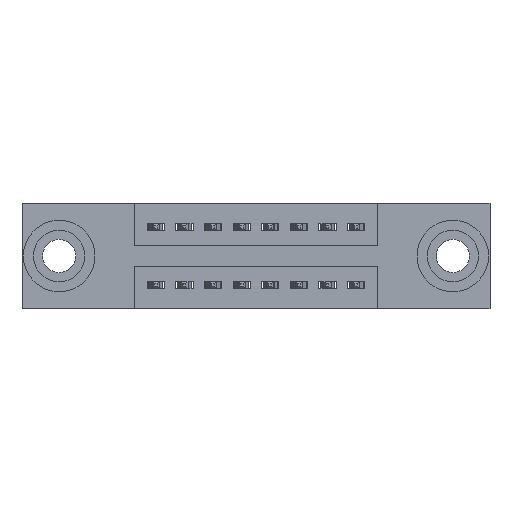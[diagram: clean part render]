
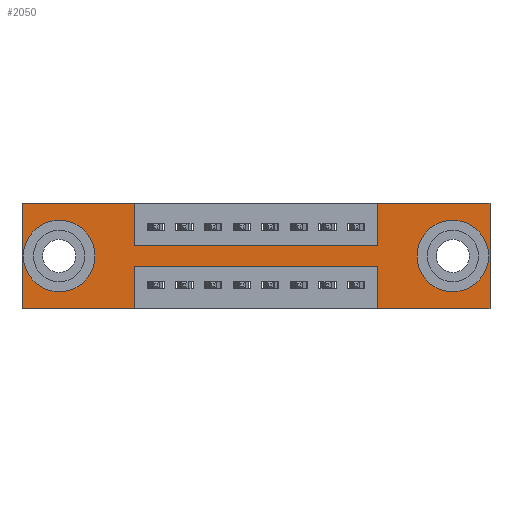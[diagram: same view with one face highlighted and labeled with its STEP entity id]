
A CAD part, front view. The second image highlights one B-rep face of the part: STEP entity #2050.
In plain terms, the highlighted planar face has unit normal (0, -1, 0).
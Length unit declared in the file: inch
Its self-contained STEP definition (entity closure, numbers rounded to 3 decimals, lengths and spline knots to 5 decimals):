
#73 = VERTEX_POINT ( 'NONE', #9574 ) ;
#88 = CARTESIAN_POINT ( 'NONE',  ( 0.13, 0., -0.263 ) ) ;
#96 = EDGE_CURVE ( 'NONE', #6298, #6497, #2246, .T. ) ;
#97 = CARTESIAN_POINT ( 'NONE',  ( 1.505, 0., -0.185 ) ) ;
#243 = EDGE_CURVE ( 'NONE', #3637, #3447, #795, .T. ) ;
#265 = VERTEX_POINT ( 'NONE', #3501 ) ;
#317 = EDGE_CURVE ( 'NONE', #73, #8299, #4881, .T. ) ;
#341 = AXIS2_PLACEMENT_3D ( 'NONE', #10581, #5446, #11437 ) ;
#378 = VERTEX_POINT ( 'NONE', #7372 ) ;
#380 = CIRCLE ( 'NONE', #341, 0.078 ) ;
#427 = EDGE_CURVE ( 'NONE', #7613, #6013, #10150, .T. ) ;
#436 = VECTOR ( 'NONE', #5695, 39.37008 ) ;
#519 = DIRECTION ( 'NONE',  ( 0., 0., -1. ) ) ;
#743 = LINE ( 'NONE', #5140, #436 ) ;
#795 = LINE ( 'NONE', #10824, #8054 ) ;
#910 = CIRCLE ( 'NONE', #2896, 0.078 ) ;
#936 = VECTOR ( 'NONE', #5049, 39.37008 ) ;
#1004 = AXIS2_PLACEMENT_3D ( 'NONE', #1729, #8076, #2676 ) ;
#1240 = ORIENTED_EDGE ( 'NONE', *, *, #7634, .F. ) ;
#1386 = ORIENTED_EDGE ( 'NONE', *, *, #8331, .T. ) ;
#1442 = CARTESIAN_POINT ( 'NONE',  ( 1.2425, 0., 0. ) ) ;
#1458 = LINE ( 'NONE', #6986, #8415 ) ;
#1478 = CIRCLE ( 'NONE', #1004, 0.078 ) ;
#1482 = DIRECTION ( 'NONE',  ( 0., 0., -1. ) ) ;
#1713 = EDGE_CURVE ( 'NONE', #10849, #4046, #7480, .T. ) ;
#1729 = CARTESIAN_POINT ( 'NONE',  ( 0.13, 0., -0.185 ) ) ;
#1845 = ORIENTED_EDGE ( 'NONE', *, *, #11431, .F. ) ;
#1887 = CARTESIAN_POINT ( 'NONE',  ( 0., 0., -0.37 ) ) ;
#1901 = CARTESIAN_POINT ( 'NONE',  ( 0.3925, 0., -0.22 ) ) ;
#2050 = ADVANCED_FACE ( 'NONE', ( #4439, #11041, #4976 ), #3816, .T. ) ;
#2130 = CARTESIAN_POINT ( 'NONE',  ( 1.2425, 0., -0.37 ) ) ;
#2155 = EDGE_CURVE ( 'NONE', #378, #265, #743, .T. ) ;
#2246 = LINE ( 'NONE', #6984, #6827 ) ;
#2374 = AXIS2_PLACEMENT_3D ( 'NONE', #97, #3207, #519 ) ;
#2391 = DIRECTION ( 'NONE',  ( 0., 0., 1. ) ) ;
#2406 = ORIENTED_EDGE ( 'NONE', *, *, #5830, .T. ) ;
#2447 = CARTESIAN_POINT ( 'NONE',  ( 1.2425, 0., 0. ) ) ;
#2641 = CARTESIAN_POINT ( 'NONE',  ( 0., 0., -0.37 ) ) ;
#2676 = DIRECTION ( 'NONE',  ( 0., 0., 1. ) ) ;
#2760 = CARTESIAN_POINT ( 'NONE',  ( 0.13, 0., -0.185 ) ) ;
#2896 = AXIS2_PLACEMENT_3D ( 'NONE', #2760, #8994, #3715 ) ;
#3080 = ORIENTED_EDGE ( 'NONE', *, *, #1713, .T. ) ;
#3207 = DIRECTION ( 'NONE',  ( 0., 1., 0. ) ) ;
#3236 = DIRECTION ( 'NONE',  ( 1., 0., 0. ) ) ;
#3447 = VERTEX_POINT ( 'NONE', #5455 ) ;
#3479 = LINE ( 'NONE', #7784, #5343 ) ;
#3501 = CARTESIAN_POINT ( 'NONE',  ( 0.3925, 0., 0. ) ) ;
#3525 = VERTEX_POINT ( 'NONE', #9854 ) ;
#3637 = VERTEX_POINT ( 'NONE', #6570 ) ;
#3715 = DIRECTION ( 'NONE',  ( 0., 0., 1. ) ) ;
#3816 = PLANE ( 'NONE',  #5268 ) ;
#4046 = VERTEX_POINT ( 'NONE', #10463 ) ;
#4229 = CARTESIAN_POINT ( 'NONE',  ( 0., 0., 0. ) ) ;
#4397 = DIRECTION ( 'NONE',  ( 0., 0., -1. ) ) ;
#4439 = FACE_BOUND ( 'NONE', #10320, .T. ) ;
#4467 = VECTOR ( 'NONE', #2391, 39.37008 ) ;
#4477 = LINE ( 'NONE', #11257, #6540 ) ;
#4527 = ORIENTED_EDGE ( 'NONE', *, *, #9853, .F. ) ;
#4642 = VECTOR ( 'NONE', #7380, 39.37008 ) ;
#4881 = LINE ( 'NONE', #5990, #6962 ) ;
#4976 = FACE_OUTER_BOUND ( 'NONE', #6169, .T. ) ;
#5018 = EDGE_CURVE ( 'NONE', #3447, #10332, #9166, .T. ) ;
#5049 = DIRECTION ( 'NONE',  ( -1., 0., 0. ) ) ;
#5063 = ORIENTED_EDGE ( 'NONE', *, *, #96, .F. ) ;
#5140 = CARTESIAN_POINT ( 'NONE',  ( 0., 0., 0. ) ) ;
#5268 = AXIS2_PLACEMENT_3D ( 'NONE', #2641, #10840, #9317 ) ;
#5343 = VECTOR ( 'NONE', #8627, 39.37008 ) ;
#5446 = DIRECTION ( 'NONE',  ( 0., 1., 0. ) ) ;
#5455 = CARTESIAN_POINT ( 'NONE',  ( 1.2425, 0., -0.37 ) ) ;
#5695 = DIRECTION ( 'NONE',  ( 1., 0., 0. ) ) ;
#5787 = ORIENTED_EDGE ( 'NONE', *, *, #8374, .T. ) ;
#5830 = EDGE_CURVE ( 'NONE', #4046, #10849, #380, .T. ) ;
#5990 = CARTESIAN_POINT ( 'NONE',  ( 0.3925, 0., -0.37 ) ) ;
#6013 = VERTEX_POINT ( 'NONE', #7481 ) ;
#6021 = ORIENTED_EDGE ( 'NONE', *, *, #243, .F. ) ;
#6169 = EDGE_LOOP ( 'NONE', ( #10918, #1845, #8825, #6021, #4527, #7926, #6978, #5063, #1240, #11039, #9654, #7009 ) ) ;
#6210 = EDGE_CURVE ( 'NONE', #6576, #378, #3479, .T. ) ;
#6298 = VERTEX_POINT ( 'NONE', #11247 ) ;
#6497 = VERTEX_POINT ( 'NONE', #8911 ) ;
#6529 = LINE ( 'NONE', #1442, #4467 ) ;
#6540 = VECTOR ( 'NONE', #4397, 39.37008 ) ;
#6570 = CARTESIAN_POINT ( 'NONE',  ( 1.635, 0., -0.37 ) ) ;
#6576 = VERTEX_POINT ( 'NONE', #1887 ) ;
#6614 = CARTESIAN_POINT ( 'NONE',  ( 1.505, 0., -0.263 ) ) ;
#6827 = VECTOR ( 'NONE', #3236, 39.37008 ) ;
#6868 = DIRECTION ( 'NONE',  ( 1., 0., 0. ) ) ;
#6962 = VECTOR ( 'NONE', #9679, 39.37008 ) ;
#6978 = ORIENTED_EDGE ( 'NONE', *, *, #8123, .F. ) ;
#6984 = CARTESIAN_POINT ( 'NONE',  ( 0.3925, 0., -0.15 ) ) ;
#6986 = CARTESIAN_POINT ( 'NONE',  ( 1.635, 0., 0. ) ) ;
#7009 = ORIENTED_EDGE ( 'NONE', *, *, #7493, .F. ) ;
#7372 = CARTESIAN_POINT ( 'NONE',  ( 0., 0., 0. ) ) ;
#7380 = DIRECTION ( 'NONE',  ( -1., 0., 0. ) ) ;
#7480 = CIRCLE ( 'NONE', #2374, 0.078 ) ;
#7481 = CARTESIAN_POINT ( 'NONE',  ( 1.635, 0., 0. ) ) ;
#7493 = EDGE_CURVE ( 'NONE', #8299, #6576, #10403, .T. ) ;
#7613 = VERTEX_POINT ( 'NONE', #2447 ) ;
#7624 = DIRECTION ( 'NONE',  ( 0., 0., 1. ) ) ;
#7634 = EDGE_CURVE ( 'NONE', #265, #6298, #4477, .T. ) ;
#7648 = VECTOR ( 'NONE', #6868, 39.37008 ) ;
#7784 = CARTESIAN_POINT ( 'NONE',  ( 0., 0., 0. ) ) ;
#7926 = ORIENTED_EDGE ( 'NONE', *, *, #427, .F. ) ;
#8054 = VECTOR ( 'NONE', #9137, 39.37008 ) ;
#8076 = DIRECTION ( 'NONE',  ( 0., 1., 0. ) ) ;
#8123 = EDGE_CURVE ( 'NONE', #6497, #7613, #6529, .T. ) ;
#8139 = EDGE_LOOP ( 'NONE', ( #1386, #5787 ) ) ;
#8299 = VERTEX_POINT ( 'NONE', #10534 ) ;
#8331 = EDGE_CURVE ( 'NONE', #3525, #10171, #1478, .T. ) ;
#8374 = EDGE_CURVE ( 'NONE', #10171, #3525, #910, .T. ) ;
#8385 = VECTOR ( 'NONE', #7624, 39.37008 ) ;
#8415 = VECTOR ( 'NONE', #1482, 39.37008 ) ;
#8627 = DIRECTION ( 'NONE',  ( 0., 0., 1. ) ) ;
#8825 = ORIENTED_EDGE ( 'NONE', *, *, #5018, .F. ) ;
#8911 = CARTESIAN_POINT ( 'NONE',  ( 1.2425, 0., -0.15 ) ) ;
#8994 = DIRECTION ( 'NONE',  ( 0., 1., 0. ) ) ;
#9137 = DIRECTION ( 'NONE',  ( -1., 0., 0. ) ) ;
#9166 = LINE ( 'NONE', #2130, #8385 ) ;
#9317 = DIRECTION ( 'NONE',  ( 0., 0., -1. ) ) ;
#9510 = LINE ( 'NONE', #1901, #4642 ) ;
#9574 = CARTESIAN_POINT ( 'NONE',  ( 0.3925, 0., -0.22 ) ) ;
#9654 = ORIENTED_EDGE ( 'NONE', *, *, #6210, .F. ) ;
#9679 = DIRECTION ( 'NONE',  ( 0., 0., -1. ) ) ;
#9853 = EDGE_CURVE ( 'NONE', #6013, #3637, #1458, .T. ) ;
#9854 = CARTESIAN_POINT ( 'NONE',  ( 0.13, 0., -0.107 ) ) ;
#10150 = LINE ( 'NONE', #4229, #7648 ) ;
#10171 = VERTEX_POINT ( 'NONE', #88 ) ;
#10320 = EDGE_LOOP ( 'NONE', ( #2406, #3080 ) ) ;
#10332 = VERTEX_POINT ( 'NONE', #11095 ) ;
#10403 = LINE ( 'NONE', #11074, #936 ) ;
#10463 = CARTESIAN_POINT ( 'NONE',  ( 1.505, 0., -0.107 ) ) ;
#10534 = CARTESIAN_POINT ( 'NONE',  ( 0.3925, 0., -0.37 ) ) ;
#10581 = CARTESIAN_POINT ( 'NONE',  ( 1.505, 0., -0.185 ) ) ;
#10824 = CARTESIAN_POINT ( 'NONE',  ( 0., 0., -0.37 ) ) ;
#10840 = DIRECTION ( 'NONE',  ( 0., -1., 0. ) ) ;
#10849 = VERTEX_POINT ( 'NONE', #6614 ) ;
#10918 = ORIENTED_EDGE ( 'NONE', *, *, #317, .F. ) ;
#11039 = ORIENTED_EDGE ( 'NONE', *, *, #2155, .F. ) ;
#11041 = FACE_BOUND ( 'NONE', #8139, .T. ) ;
#11074 = CARTESIAN_POINT ( 'NONE',  ( 0., 0., -0.37 ) ) ;
#11095 = CARTESIAN_POINT ( 'NONE',  ( 1.2425, 0., -0.22 ) ) ;
#11247 = CARTESIAN_POINT ( 'NONE',  ( 0.3925, 0., -0.15 ) ) ;
#11257 = CARTESIAN_POINT ( 'NONE',  ( 0.3925, 0., 0. ) ) ;
#11431 = EDGE_CURVE ( 'NONE', #10332, #73, #9510, .T. ) ;
#11437 = DIRECTION ( 'NONE',  ( 0., 0., -1. ) ) ;
